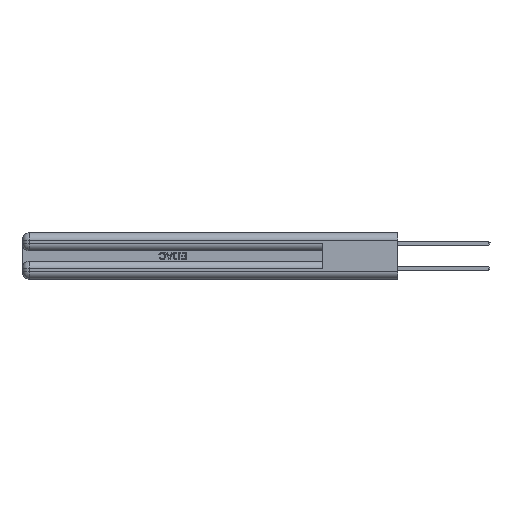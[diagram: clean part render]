
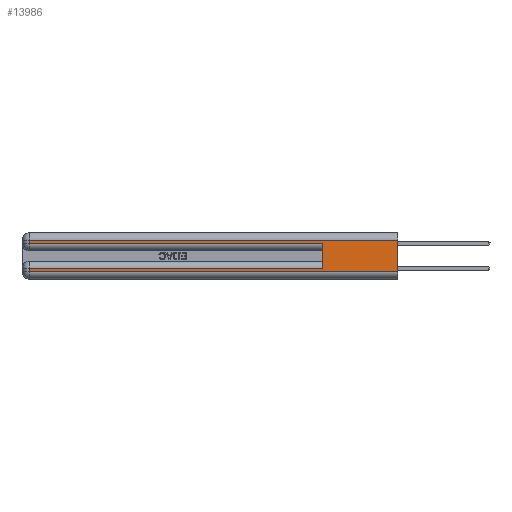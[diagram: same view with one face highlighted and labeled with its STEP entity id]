
A CAD part, left-side view. The second image highlights one B-rep face of the part: STEP entity #13986.
In plain terms, the highlighted planar face has unit normal (-1, 0, 0).
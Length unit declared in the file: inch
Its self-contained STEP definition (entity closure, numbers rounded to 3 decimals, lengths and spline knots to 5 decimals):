
#9 = VECTOR ( 'NONE', #13125, 39.37008 ) ;
#412 = DIRECTION ( 'NONE',  ( 0., 0., -1. ) ) ;
#1643 = DIRECTION ( 'NONE',  ( 0., 1., 0. ) ) ;
#2423 = VECTOR ( 'NONE', #43803, 39.37008 ) ;
#3106 = VERTEX_POINT ( 'NONE', #9981 ) ;
#5497 = VERTEX_POINT ( 'NONE', #47322 ) ;
#6590 = ORIENTED_EDGE ( 'NONE', *, *, #24859, .T. ) ;
#7093 = EDGE_CURVE ( 'NONE', #25272, #27294, #49258, .T. ) ;
#7888 = LINE ( 'NONE', #32439, #2423 ) ;
#8771 = VERTEX_POINT ( 'NONE', #41866 ) ;
#8991 = CARTESIAN_POINT ( 'NONE',  ( 0., 0., 0.31 ) ) ;
#9981 = CARTESIAN_POINT ( 'NONE',  ( 0., 0., 0.06 ) ) ;
#10679 = EDGE_CURVE ( 'NONE', #5497, #3106, #13382, .T. ) ;
#13125 = DIRECTION ( 'NONE',  ( 0., 1., 0. ) ) ;
#13382 = LINE ( 'NONE', #35891, #34587 ) ;
#13986 = ADVANCED_FACE ( 'NONE', ( #14858 ), #47148, .F. ) ;
#14011 = LINE ( 'NONE', #44345, #9 ) ;
#14858 = FACE_OUTER_BOUND ( 'NONE', #41046, .T. ) ;
#15846 = LINE ( 'NONE', #8991, #31613 ) ;
#17579 = DIRECTION ( 'NONE',  ( 1., 0., 0. ) ) ;
#19053 = EDGE_CURVE ( 'NONE', #25272, #8771, #14011, .T. ) ;
#19064 = CARTESIAN_POINT ( 'NONE',  ( 0., 2.94, 0.06 ) ) ;
#20891 = VERTEX_POINT ( 'NONE', #48408 ) ;
#21979 = CARTESIAN_POINT ( 'NONE',  ( 0., 0.6, 0.085 ) ) ;
#22519 = VECTOR ( 'NONE', #41857, 39.37008 ) ;
#22690 = LINE ( 'NONE', #32135, #42610 ) ;
#22917 = DIRECTION ( 'NONE',  ( 0., 0., 1. ) ) ;
#23851 = CARTESIAN_POINT ( 'NONE',  ( 0., 2.94, 0.37 ) ) ;
#24566 = EDGE_CURVE ( 'NONE', #5497, #20891, #15846, .T. ) ;
#24859 = EDGE_CURVE ( 'NONE', #37544, #27294, #37061, .T. ) ;
#25272 = VERTEX_POINT ( 'NONE', #21979 ) ;
#25900 = ORIENTED_EDGE ( 'NONE', *, *, #46022, .T. ) ;
#26247 = CARTESIAN_POINT ( 'NONE',  ( 0., 0., 0.285 ) ) ;
#27294 = VERTEX_POINT ( 'NONE', #32792 ) ;
#28310 = ORIENTED_EDGE ( 'NONE', *, *, #42562, .T. ) ;
#29806 = VECTOR ( 'NONE', #22917, 39.37008 ) ;
#30462 = VECTOR ( 'NONE', #412, 39.37008 ) ;
#31257 = AXIS2_PLACEMENT_3D ( 'NONE', #41201, #17579, #39139 ) ;
#31613 = VECTOR ( 'NONE', #1643, 39.37008 ) ;
#32135 = CARTESIAN_POINT ( 'NONE',  ( 0., 0., 0.06 ) ) ;
#32439 = CARTESIAN_POINT ( 'NONE',  ( 0., 2.94, 0.37 ) ) ;
#32792 = CARTESIAN_POINT ( 'NONE',  ( 0., 0.6, 0.285 ) ) ;
#34587 = VECTOR ( 'NONE', #39796, 39.37008 ) ;
#35162 = ORIENTED_EDGE ( 'NONE', *, *, #39216, .T. ) ;
#35678 = VERTEX_POINT ( 'NONE', #19064 ) ;
#35891 = CARTESIAN_POINT ( 'NONE',  ( 0., 0., 0.37 ) ) ;
#37061 = LINE ( 'NONE', #26247, #22519 ) ;
#37544 = VERTEX_POINT ( 'NONE', #41801 ) ;
#39076 = ORIENTED_EDGE ( 'NONE', *, *, #10679, .F. ) ;
#39139 = DIRECTION ( 'NONE',  ( 0., 0., -1. ) ) ;
#39216 = EDGE_CURVE ( 'NONE', #20891, #37544, #7888, .T. ) ;
#39796 = DIRECTION ( 'NONE',  ( 0., 0., -1. ) ) ;
#40798 = LINE ( 'NONE', #23851, #30462 ) ;
#41046 = EDGE_LOOP ( 'NONE', ( #39076, #43878, #35162, #6590, #42636, #48971, #25900, #28310 ) ) ;
#41201 = CARTESIAN_POINT ( 'NONE',  ( 0., 0., 0.37 ) ) ;
#41801 = CARTESIAN_POINT ( 'NONE',  ( 0., 2.94, 0.285 ) ) ;
#41857 = DIRECTION ( 'NONE',  ( 0., -1., 0. ) ) ;
#41866 = CARTESIAN_POINT ( 'NONE',  ( 0., 2.94, 0.085 ) ) ;
#42439 = CARTESIAN_POINT ( 'NONE',  ( 0., 0.6, 0.145 ) ) ;
#42562 = EDGE_CURVE ( 'NONE', #35678, #3106, #22690, .T. ) ;
#42610 = VECTOR ( 'NONE', #44167, 39.37008 ) ;
#42636 = ORIENTED_EDGE ( 'NONE', *, *, #7093, .F. ) ;
#43803 = DIRECTION ( 'NONE',  ( 0., 0., -1. ) ) ;
#43878 = ORIENTED_EDGE ( 'NONE', *, *, #24566, .T. ) ;
#44167 = DIRECTION ( 'NONE',  ( 0., -1., 0. ) ) ;
#44345 = CARTESIAN_POINT ( 'NONE',  ( 0., 0., 0.085 ) ) ;
#46022 = EDGE_CURVE ( 'NONE', #8771, #35678, #40798, .T. ) ;
#47148 = PLANE ( 'NONE',  #31257 ) ;
#47322 = CARTESIAN_POINT ( 'NONE',  ( 0., 0., 0.31 ) ) ;
#48408 = CARTESIAN_POINT ( 'NONE',  ( 0., 2.94, 0.31 ) ) ;
#48971 = ORIENTED_EDGE ( 'NONE', *, *, #19053, .T. ) ;
#49258 = LINE ( 'NONE', #42439, #29806 ) ;
